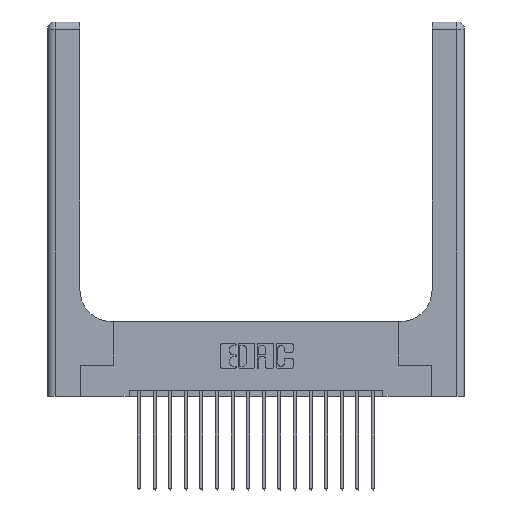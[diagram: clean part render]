
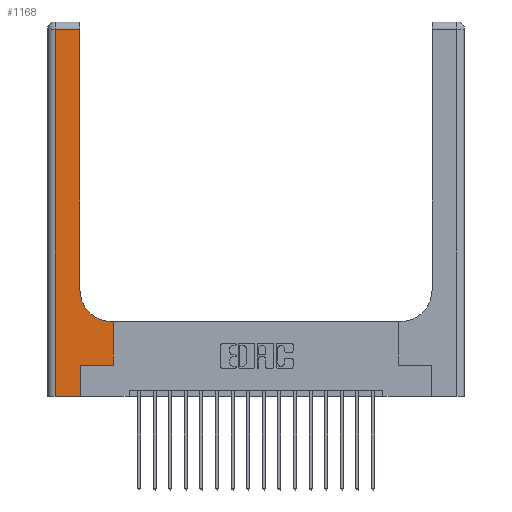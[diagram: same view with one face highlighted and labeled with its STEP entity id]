
A CAD part, top view. The second image highlights one B-rep face of the part: STEP entity #1168.
In plain terms, the highlighted planar face has unit normal (0, 0, 1).
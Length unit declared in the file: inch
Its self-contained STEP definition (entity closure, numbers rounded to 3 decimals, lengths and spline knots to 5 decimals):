
#199 = VECTOR ( 'NONE', #362, 39.37008 ) ;
#362 = DIRECTION ( 'NONE',  ( -1., 0., 0. ) ) ;
#480 = VECTOR ( 'NONE', #861, 39.37008 ) ;
#549 = CARTESIAN_POINT ( 'NONE',  ( 0.528, 0.6, 0.37 ) ) ;
#681 = CARTESIAN_POINT ( 'NONE',  ( 0., 3., 0.37 ) ) ;
#861 = DIRECTION ( 'NONE',  ( 0., 1., 0. ) ) ;
#898 = VECTOR ( 'NONE', #3312, 39.37008 ) ;
#1159 = VERTEX_POINT ( 'NONE', #3697 ) ;
#1168 = ADVANCED_FACE ( 'NONE', ( #1517 ), #9515, .F. ) ;
#1430 = EDGE_CURVE ( 'NONE', #4798, #8800, #1498, .T. ) ;
#1498 = LINE ( 'NONE', #6425, #3142 ) ;
#1517 = FACE_OUTER_BOUND ( 'NONE', #4567, .T. ) ;
#2252 = ORIENTED_EDGE ( 'NONE', *, *, #9750, .T. ) ;
#2422 = CIRCLE ( 'NONE', #4829, 0.25 ) ;
#2753 = VERTEX_POINT ( 'NONE', #15500 ) ;
#2996 = LINE ( 'NONE', #18860, #16607 ) ;
#3125 = CARTESIAN_POINT ( 'NONE',  ( 0.265, 0., 0.37 ) ) ;
#3142 = VECTOR ( 'NONE', #13704, 39.37008 ) ;
#3180 = CARTESIAN_POINT ( 'NONE',  ( 0.26, 0.85, 0.37 ) ) ;
#3312 = DIRECTION ( 'NONE',  ( 1., 0., 0. ) ) ;
#3371 = EDGE_CURVE ( 'NONE', #18159, #2753, #14626, .T. ) ;
#3433 = CARTESIAN_POINT ( 'NONE',  ( 0.265, 0.25, 0.37 ) ) ;
#3576 = DIRECTION ( 'NONE',  ( 0., 1., 0. ) ) ;
#3697 = CARTESIAN_POINT ( 'NONE',  ( 0.06, 2.94, 0.37 ) ) ;
#3862 = AXIS2_PLACEMENT_3D ( 'NONE', #681, #9645, #11167 ) ;
#4450 = EDGE_CURVE ( 'NONE', #1159, #4798, #5553, .T. ) ;
#4567 = EDGE_LOOP ( 'NONE', ( #18033, #16487, #10093, #6884, #5245, #6374, #17598, #16794, #2252 ) ) ;
#4798 = VERTEX_POINT ( 'NONE', #17441 ) ;
#4808 = CARTESIAN_POINT ( 'NONE',  ( 0.51, 0.85, 0.37 ) ) ;
#4829 = AXIS2_PLACEMENT_3D ( 'NONE', #4808, #9115, #13756 ) ;
#4846 = LINE ( 'NONE', #3433, #898 ) ;
#5037 = EDGE_CURVE ( 'NONE', #16111, #13675, #14787, .T. ) ;
#5075 = EDGE_CURVE ( 'NONE', #17531, #16033, #4846, .T. ) ;
#5245 = ORIENTED_EDGE ( 'NONE', *, *, #15439, .T. ) ;
#5340 = CARTESIAN_POINT ( 'NONE',  ( 0.26, 3., 0.37 ) ) ;
#5553 = LINE ( 'NONE', #7847, #16663 ) ;
#6374 = ORIENTED_EDGE ( 'NONE', *, *, #5075, .T. ) ;
#6425 = CARTESIAN_POINT ( 'NONE',  ( 0., 0., 0.37 ) ) ;
#6884 = ORIENTED_EDGE ( 'NONE', *, *, #1430, .T. ) ;
#7605 = VECTOR ( 'NONE', #3576, 39.37008 ) ;
#7753 = CARTESIAN_POINT ( 'NONE',  ( 0.528, 0.25, 0.37 ) ) ;
#7847 = CARTESIAN_POINT ( 'NONE',  ( 0.06, 3., 0.37 ) ) ;
#8345 = CARTESIAN_POINT ( 'NONE',  ( 0.528, 0.25, 0.37 ) ) ;
#8800 = VERTEX_POINT ( 'NONE', #3125 ) ;
#9115 = DIRECTION ( 'NONE',  ( 0., 0., -1. ) ) ;
#9515 = PLANE ( 'NONE',  #3862 ) ;
#9556 = DIRECTION ( 'NONE',  ( 0., -1., 0. ) ) ;
#9645 = DIRECTION ( 'NONE',  ( 0., 0., -1. ) ) ;
#9750 = EDGE_CURVE ( 'NONE', #13675, #18159, #2422, .T. ) ;
#10093 = ORIENTED_EDGE ( 'NONE', *, *, #4450, .T. ) ;
#10889 = CARTESIAN_POINT ( 'NONE',  ( 0.265, 0., 0.37 ) ) ;
#11167 = DIRECTION ( 'NONE',  ( -1., 0., 0. ) ) ;
#12411 = EDGE_CURVE ( 'NONE', #16033, #16111, #18020, .T. ) ;
#12717 = DIRECTION ( 'NONE',  ( 0., 1., 0. ) ) ;
#13675 = VERTEX_POINT ( 'NONE', #17927 ) ;
#13704 = DIRECTION ( 'NONE',  ( 1., 0., 0. ) ) ;
#13756 = DIRECTION ( 'NONE',  ( 1., 0., 0. ) ) ;
#14626 = LINE ( 'NONE', #5340, #480 ) ;
#14787 = LINE ( 'NONE', #18202, #199 ) ;
#15135 = CARTESIAN_POINT ( 'NONE',  ( 0.265, 0.25, 0.37 ) ) ;
#15439 = EDGE_CURVE ( 'NONE', #8800, #17531, #18214, .T. ) ;
#15500 = CARTESIAN_POINT ( 'NONE',  ( 0.26, 2.94, 0.37 ) ) ;
#15769 = EDGE_CURVE ( 'NONE', #2753, #1159, #2996, .T. ) ;
#15970 = DIRECTION ( 'NONE',  ( -1., 0., 0. ) ) ;
#16033 = VERTEX_POINT ( 'NONE', #7753 ) ;
#16111 = VERTEX_POINT ( 'NONE', #549 ) ;
#16487 = ORIENTED_EDGE ( 'NONE', *, *, #15769, .T. ) ;
#16607 = VECTOR ( 'NONE', #15970, 39.37008 ) ;
#16663 = VECTOR ( 'NONE', #9556, 39.37008 ) ;
#16794 = ORIENTED_EDGE ( 'NONE', *, *, #5037, .T. ) ;
#17441 = CARTESIAN_POINT ( 'NONE',  ( 0.06, 0., 0.37 ) ) ;
#17531 = VERTEX_POINT ( 'NONE', #15135 ) ;
#17598 = ORIENTED_EDGE ( 'NONE', *, *, #12411, .T. ) ;
#17927 = CARTESIAN_POINT ( 'NONE',  ( 0.51, 0.6, 0.37 ) ) ;
#18020 = LINE ( 'NONE', #8345, #18255 ) ;
#18033 = ORIENTED_EDGE ( 'NONE', *, *, #3371, .T. ) ;
#18159 = VERTEX_POINT ( 'NONE', #3180 ) ;
#18202 = CARTESIAN_POINT ( 'NONE',  ( 0.26, 0.6, 0.37 ) ) ;
#18214 = LINE ( 'NONE', #10889, #7605 ) ;
#18255 = VECTOR ( 'NONE', #12717, 39.37008 ) ;
#18860 = CARTESIAN_POINT ( 'NONE',  ( 0., 2.94, 0.37 ) ) ;
